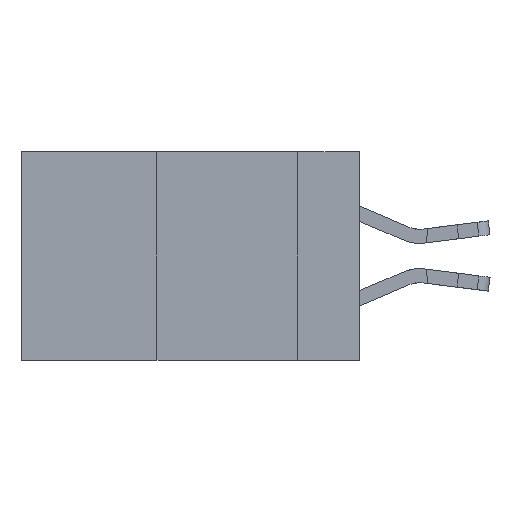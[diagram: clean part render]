
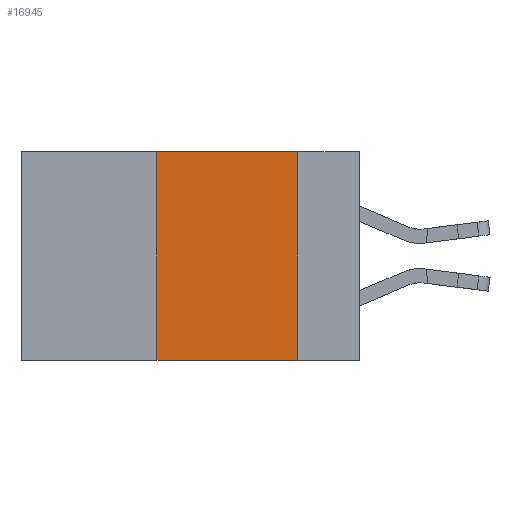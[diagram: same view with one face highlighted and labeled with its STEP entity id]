
A CAD part, left-side view. The second image highlights one B-rep face of the part: STEP entity #16945.
In plain terms, the highlighted planar face has unit normal (-1, 0, 0).
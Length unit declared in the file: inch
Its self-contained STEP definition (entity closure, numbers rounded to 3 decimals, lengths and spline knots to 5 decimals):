
#794 = EDGE_CURVE ( 'NONE', #3102, #13032, #10756, .T. ) ;
#959 = ORIENTED_EDGE ( 'NONE', *, *, #794, .F. ) ;
#998 = LINE ( 'NONE', #14926, #14814 ) ;
#1698 = EDGE_CURVE ( 'NONE', #13032, #16932, #14351, .T. ) ;
#1940 = DIRECTION ( 'NONE',  ( 0., 0., 1. ) ) ;
#1962 = CARTESIAN_POINT ( 'NONE',  ( 0., 0.36, 0. ) ) ;
#2126 = ORIENTED_EDGE ( 'NONE', *, *, #15022, .T. ) ;
#2215 = CARTESIAN_POINT ( 'NONE',  ( 0., 0.36, 0. ) ) ;
#3102 = VERTEX_POINT ( 'NONE', #12840 ) ;
#3342 = VECTOR ( 'NONE', #17462, 39.37008 ) ;
#3749 = DIRECTION ( 'NONE',  ( 0., 0., -1. ) ) ;
#4197 = AXIS2_PLACEMENT_3D ( 'NONE', #15985, #12023, #3749 ) ;
#4249 = VERTEX_POINT ( 'NONE', #11678 ) ;
#4454 = FACE_OUTER_BOUND ( 'NONE', #11291, .T. ) ;
#4590 = EDGE_CURVE ( 'NONE', #16932, #4249, #17396, .T. ) ;
#5137 = CARTESIAN_POINT ( 'NONE',  ( 0., 0.11, 0. ) ) ;
#6577 = VECTOR ( 'NONE', #10671, 39.37008 ) ;
#7926 = PLANE ( 'NONE',  #4197 ) ;
#8000 = ORIENTED_EDGE ( 'NONE', *, *, #4590, .F. ) ;
#10671 = DIRECTION ( 'NONE',  ( 0., 0., -1. ) ) ;
#10756 = LINE ( 'NONE', #1962, #17511 ) ;
#10850 = CARTESIAN_POINT ( 'NONE',  ( 0., 0.11, 0. ) ) ;
#11012 = ORIENTED_EDGE ( 'NONE', *, *, #1698, .F. ) ;
#11291 = EDGE_LOOP ( 'NONE', ( #8000, #11012, #959, #2126 ) ) ;
#11678 = CARTESIAN_POINT ( 'NONE',  ( 0., 0.11, -0.37 ) ) ;
#12023 = DIRECTION ( 'NONE',  ( 1., 0., 0. ) ) ;
#12296 = CARTESIAN_POINT ( 'NONE',  ( 0., 0.6, 0. ) ) ;
#12840 = CARTESIAN_POINT ( 'NONE',  ( 0., 0.36, -0.37 ) ) ;
#13032 = VERTEX_POINT ( 'NONE', #2215 ) ;
#14351 = LINE ( 'NONE', #12296, #3342 ) ;
#14814 = VECTOR ( 'NONE', #16253, 39.37008 ) ;
#14926 = CARTESIAN_POINT ( 'NONE',  ( 0., 0.6, -0.37 ) ) ;
#15022 = EDGE_CURVE ( 'NONE', #3102, #4249, #998, .T. ) ;
#15985 = CARTESIAN_POINT ( 'NONE',  ( 0., 0.6, 0. ) ) ;
#16253 = DIRECTION ( 'NONE',  ( 0., -1., 0. ) ) ;
#16932 = VERTEX_POINT ( 'NONE', #5137 ) ;
#16945 = ADVANCED_FACE ( 'NONE', ( #4454 ), #7926, .F. ) ;
#17396 = LINE ( 'NONE', #10850, #6577 ) ;
#17462 = DIRECTION ( 'NONE',  ( 0., -1., 0. ) ) ;
#17511 = VECTOR ( 'NONE', #1940, 39.37008 ) ;
